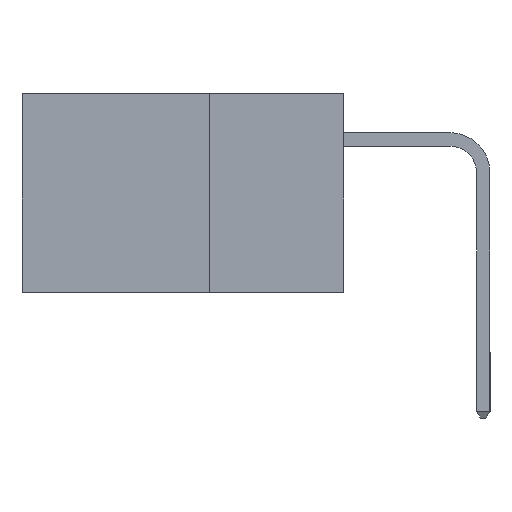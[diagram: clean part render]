
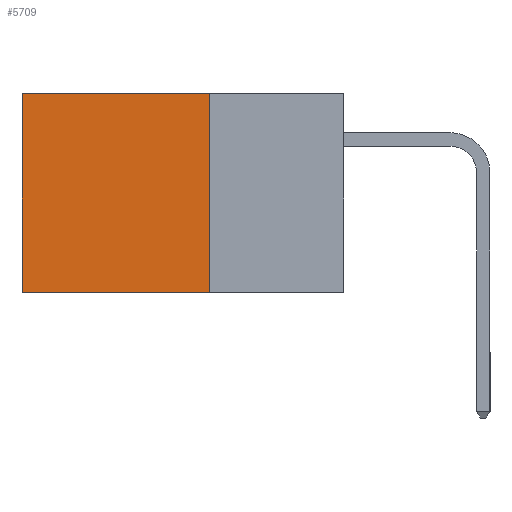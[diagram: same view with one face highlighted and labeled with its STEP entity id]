
A CAD part, left-side view. The second image highlights one B-rep face of the part: STEP entity #5709.
In plain terms, the highlighted planar face has unit normal (-1, 0, 0).
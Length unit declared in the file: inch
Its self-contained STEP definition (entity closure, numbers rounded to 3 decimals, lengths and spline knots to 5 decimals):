
#653 = ORIENTED_EDGE ( 'NONE', *, *, #758, .F. ) ;
#758 = EDGE_CURVE ( 'NONE', #11222, #16744, #13376, .T. ) ;
#874 = EDGE_CURVE ( 'NONE', #12607, #11222, #15163, .T. ) ;
#1053 = CARTESIAN_POINT ( 'NONE',  ( 0.2615, 0.25, -0.37 ) ) ;
#1172 = FACE_OUTER_BOUND ( 'NONE', #24603, .T. ) ;
#1716 = AXIS2_PLACEMENT_3D ( 'NONE', #1053, #3235, #14624 ) ;
#1858 = DIRECTION ( 'NONE',  ( 0., 1., 0. ) ) ;
#2987 = CARTESIAN_POINT ( 'NONE',  ( 0.2615, 0.25, 0. ) ) ;
#3235 = DIRECTION ( 'NONE',  ( 1., 0., 0. ) ) ;
#3918 = CARTESIAN_POINT ( 'NONE',  ( 0.2615, 0.25, -0.37 ) ) ;
#3968 = VECTOR ( 'NONE', #16688, 39.37008 ) ;
#4122 = CARTESIAN_POINT ( 'NONE',  ( 0.2615, 0.6, 0. ) ) ;
#5709 = ADVANCED_FACE ( 'NONE', ( #1172 ), #7093, .F. ) ;
#7093 = PLANE ( 'NONE',  #1716 ) ;
#7506 = CARTESIAN_POINT ( 'NONE',  ( 0.2615, 0.25, -0.37 ) ) ;
#7574 = CARTESIAN_POINT ( 'NONE',  ( 0.2615, 0.25, 0. ) ) ;
#8406 = CARTESIAN_POINT ( 'NONE',  ( 0.2615, 0.6, -0.37 ) ) ;
#10329 = LINE ( 'NONE', #8406, #17243 ) ;
#11222 = VERTEX_POINT ( 'NONE', #13736 ) ;
#12007 = VECTOR ( 'NONE', #1858, 39.37008 ) ;
#12607 = VERTEX_POINT ( 'NONE', #7574 ) ;
#13376 = LINE ( 'NONE', #3918, #12007 ) ;
#13736 = CARTESIAN_POINT ( 'NONE',  ( 0.2615, 0.25, -0.37 ) ) ;
#14026 = VERTEX_POINT ( 'NONE', #4122 ) ;
#14624 = DIRECTION ( 'NONE',  ( 0., 0., -1. ) ) ;
#15077 = EDGE_CURVE ( 'NONE', #12607, #14026, #20512, .T. ) ;
#15163 = LINE ( 'NONE', #7506, #21877 ) ;
#15698 = DIRECTION ( 'NONE',  ( 0., 0., -1. ) ) ;
#16095 = DIRECTION ( 'NONE',  ( 0., 0., -1. ) ) ;
#16373 = ORIENTED_EDGE ( 'NONE', *, *, #874, .F. ) ;
#16688 = DIRECTION ( 'NONE',  ( 0., 1., 0. ) ) ;
#16744 = VERTEX_POINT ( 'NONE', #22293 ) ;
#17243 = VECTOR ( 'NONE', #16095, 39.37008 ) ;
#19021 = ORIENTED_EDGE ( 'NONE', *, *, #15077, .T. ) ;
#20512 = LINE ( 'NONE', #2987, #3968 ) ;
#21877 = VECTOR ( 'NONE', #15698, 39.37008 ) ;
#22293 = CARTESIAN_POINT ( 'NONE',  ( 0.2615, 0.6, -0.37 ) ) ;
#23920 = ORIENTED_EDGE ( 'NONE', *, *, #24600, .T. ) ;
#24600 = EDGE_CURVE ( 'NONE', #14026, #16744, #10329, .T. ) ;
#24603 = EDGE_LOOP ( 'NONE', ( #23920, #653, #16373, #19021 ) ) ;
